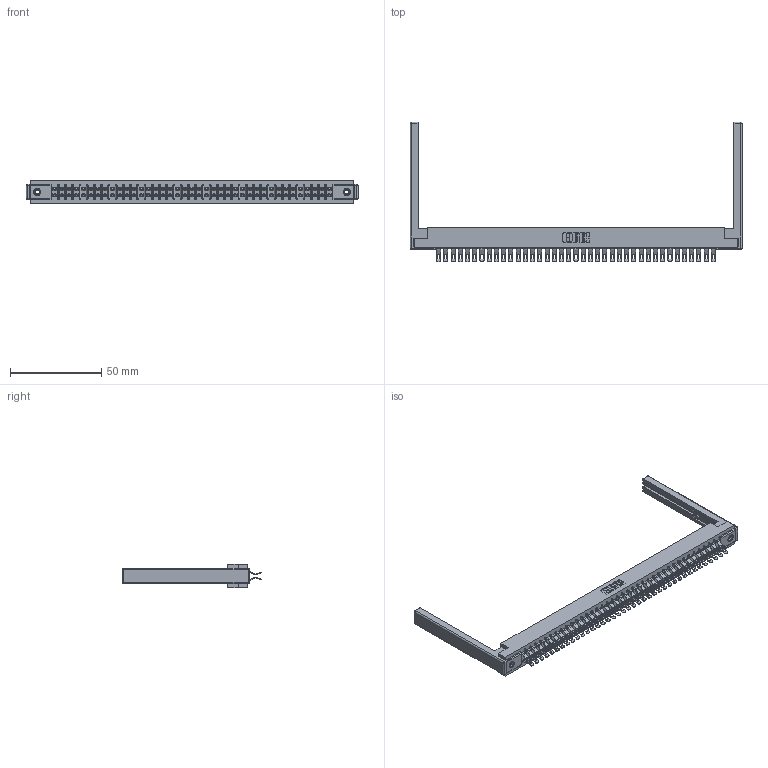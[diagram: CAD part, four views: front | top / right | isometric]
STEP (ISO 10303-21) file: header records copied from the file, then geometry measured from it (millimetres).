
FILE_DESCRIPTION (( 'STEP AP203' ), '1' );
FILE_NAME ('307-078-555-268.STEP', '2019-09-06T23:05:21', ( '' ), ( '' ), 'SwSTEP 2.0', 'SolidWorks 2016', '' );
FILE_SCHEMA (( 'CONFIG_CONTROL_DESIGN' ));
Length unit declared in the file: inch
Products named in the file (5): 307-290-001_555; 307-220-068; 307-078-555-268; 307 Part_.156 Dia Mounting Holes; 345-250-001_345-250-001-102
Assembly tree (83 placements, depth 2):
  307-078-555-268
    307 Part_.156 Dia Mounting Holes
    307-290-001_555  x78
    307-220-068  x2
    345-250-001_345-250-001-102  x2
Bounding box: 181.97 x 76.71 x 12.7 mm (x, y, z)
Volume: 23941.6 mm3; surface area: 29145.3 mm2
Topology: 83 solids, 83 shells, 5070 faces, 14831 edges, 9654 vertices
Faces by surface type: plane 2810, cylinder 2156, sphere 88, cone 12, torus 4
Entity records: 38348 total; most frequent: CARTESIAN_POINT 6256, ORIENTED_EDGE 6194, DIRECTION 6151, EDGE_CURVE 3097, LINE 2361, VECTOR 2361, VERTEX_POINT 2000, AXIS2_PLACEMENT_3D 1895
